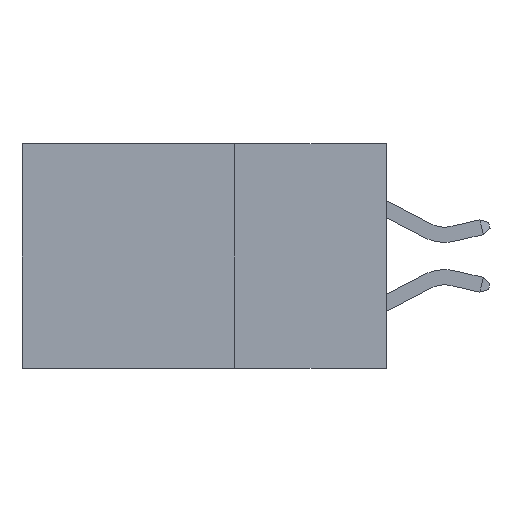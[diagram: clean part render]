
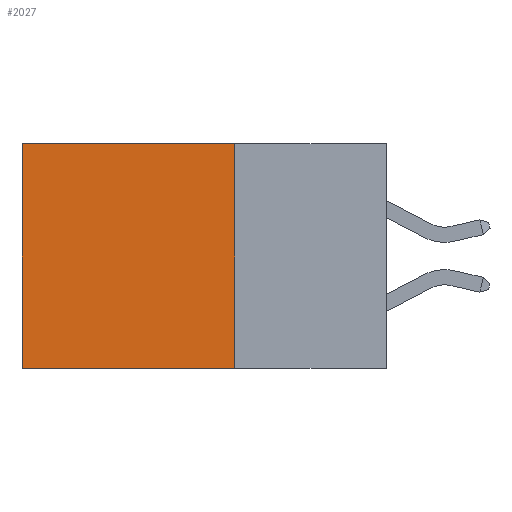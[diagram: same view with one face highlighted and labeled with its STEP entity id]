
A CAD part, left-side view. The second image highlights one B-rep face of the part: STEP entity #2027.
In plain terms, the highlighted planar face has unit normal (-1, 0, 0).
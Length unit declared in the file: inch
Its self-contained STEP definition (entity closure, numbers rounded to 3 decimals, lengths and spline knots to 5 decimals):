
#184 = EDGE_CURVE ( 'NONE', #1194, #19931, #6189, .T. ) ;
#549 = ORIENTED_EDGE ( 'NONE', *, *, #184, .T. ) ;
#1066 = DIRECTION ( 'NONE',  ( 1., 0., 0. ) ) ;
#1194 = VERTEX_POINT ( 'NONE', #17150 ) ;
#1395 = VERTEX_POINT ( 'NONE', #22099 ) ;
#2027 = ADVANCED_FACE ( 'NONE', ( #23058 ), #12709, .F. ) ;
#2137 = CARTESIAN_POINT ( 'NONE',  ( 0.2615, 0.6, -0.37 ) ) ;
#4238 = LINE ( 'NONE', #14159, #24078 ) ;
#4483 = EDGE_LOOP ( 'NONE', ( #549, #24762, #16592, #19813 ) ) ;
#4995 = VECTOR ( 'NONE', #18899, 39.37008 ) ;
#5218 = EDGE_CURVE ( 'NONE', #9670, #19931, #12945, .T. ) ;
#5295 = CARTESIAN_POINT ( 'NONE',  ( 0.2615, 0.25, -0.37 ) ) ;
#6189 = LINE ( 'NONE', #2137, #20675 ) ;
#6824 = CARTESIAN_POINT ( 'NONE',  ( 0.2615, 0.25, 0. ) ) ;
#7079 = LINE ( 'NONE', #6824, #4995 ) ;
#9019 = DIRECTION ( 'NONE',  ( 0., 0., -1. ) ) ;
#9670 = VERTEX_POINT ( 'NONE', #5295 ) ;
#12709 = PLANE ( 'NONE',  #15758 ) ;
#12945 = LINE ( 'NONE', #16930, #20790 ) ;
#14159 = CARTESIAN_POINT ( 'NONE',  ( 0.2615, 0.25, -0.37 ) ) ;
#15005 = CARTESIAN_POINT ( 'NONE',  ( 0.2615, 0.25, -0.37 ) ) ;
#15758 = AXIS2_PLACEMENT_3D ( 'NONE', #15005, #1066, #9019 ) ;
#16046 = EDGE_CURVE ( 'NONE', #1395, #1194, #7079, .T. ) ;
#16075 = DIRECTION ( 'NONE',  ( 0., 0., -1. ) ) ;
#16592 = ORIENTED_EDGE ( 'NONE', *, *, #22480, .F. ) ;
#16930 = CARTESIAN_POINT ( 'NONE',  ( 0.2615, 0.25, -0.37 ) ) ;
#17150 = CARTESIAN_POINT ( 'NONE',  ( 0.2615, 0.6, 0. ) ) ;
#17909 = DIRECTION ( 'NONE',  ( 0., 0., -1. ) ) ;
#18899 = DIRECTION ( 'NONE',  ( 0., 1., 0. ) ) ;
#19813 = ORIENTED_EDGE ( 'NONE', *, *, #16046, .T. ) ;
#19931 = VERTEX_POINT ( 'NONE', #22872 ) ;
#20675 = VECTOR ( 'NONE', #16075, 39.37008 ) ;
#20790 = VECTOR ( 'NONE', #24876, 39.37008 ) ;
#22099 = CARTESIAN_POINT ( 'NONE',  ( 0.2615, 0.25, 0. ) ) ;
#22480 = EDGE_CURVE ( 'NONE', #1395, #9670, #4238, .T. ) ;
#22872 = CARTESIAN_POINT ( 'NONE',  ( 0.2615, 0.6, -0.37 ) ) ;
#23058 = FACE_OUTER_BOUND ( 'NONE', #4483, .T. ) ;
#24078 = VECTOR ( 'NONE', #17909, 39.37008 ) ;
#24762 = ORIENTED_EDGE ( 'NONE', *, *, #5218, .F. ) ;
#24876 = DIRECTION ( 'NONE',  ( 0., 1., 0. ) ) ;
